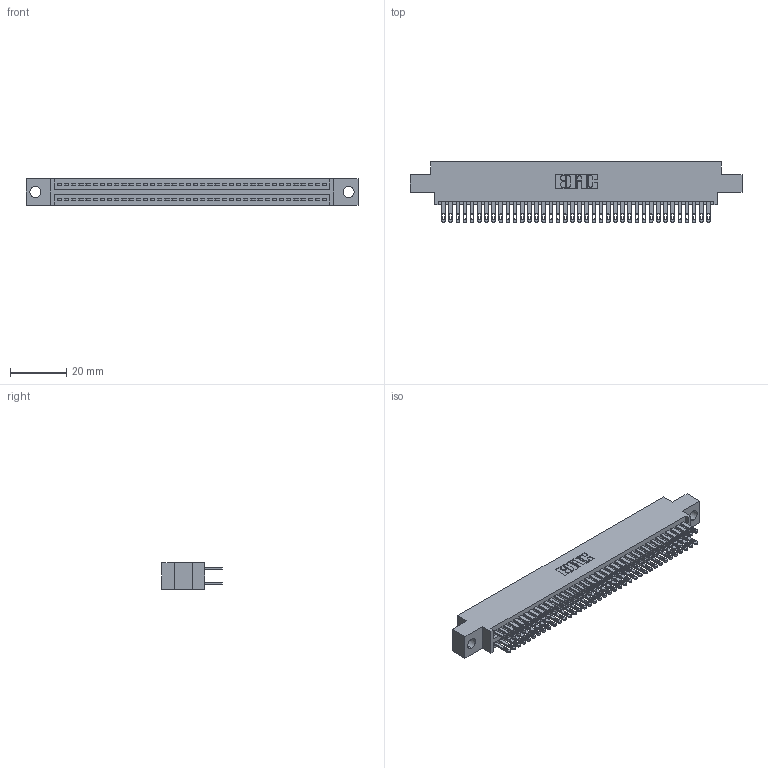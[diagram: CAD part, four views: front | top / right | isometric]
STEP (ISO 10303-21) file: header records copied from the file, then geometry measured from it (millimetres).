
FILE_DESCRIPTION (( 'STEP AP203' ), '1' );
FILE_NAME ('345-076-500-804.STEP', '2018-10-02T14:50:52', ( '' ), ( '' ), 'SwSTEP 2.0', 'SolidWorks 2016', '' );
FILE_SCHEMA (( 'CONFIG_CONTROL_DESIGN' ));
Length unit declared in the file: inch
Products named in the file (3): 345 Part_0.170 Offset - 0.156 Dia-TH; 345-076-500-804; 345-292-001_345-293-100
Assembly tree (77 placements, depth 2):
  345-076-500-804
    345 Part_0.170 Offset - 0.156 Dia-TH
    345-292-001_345-293-100  x76
Bounding box: 117.73 x 21.51 x 9.4 mm (x, y, z)
Volume: 11430.2 mm3; surface area: 17552.1 mm2
Topology: 77 solids, 77 shells, 3626 faces, 11069 edges, 7378 vertices
Faces by surface type: plane 2136, cylinder 1490
Entity records: 30419 total; most frequent: CARTESIAN_POINT 5104, ORIENTED_EDGE 5038, DIRECTION 4507, EDGE_CURVE 2519, VECTOR 2231, LINE 2231, VERTEX_POINT 1678, AXIS2_PLACEMENT_3D 1138
